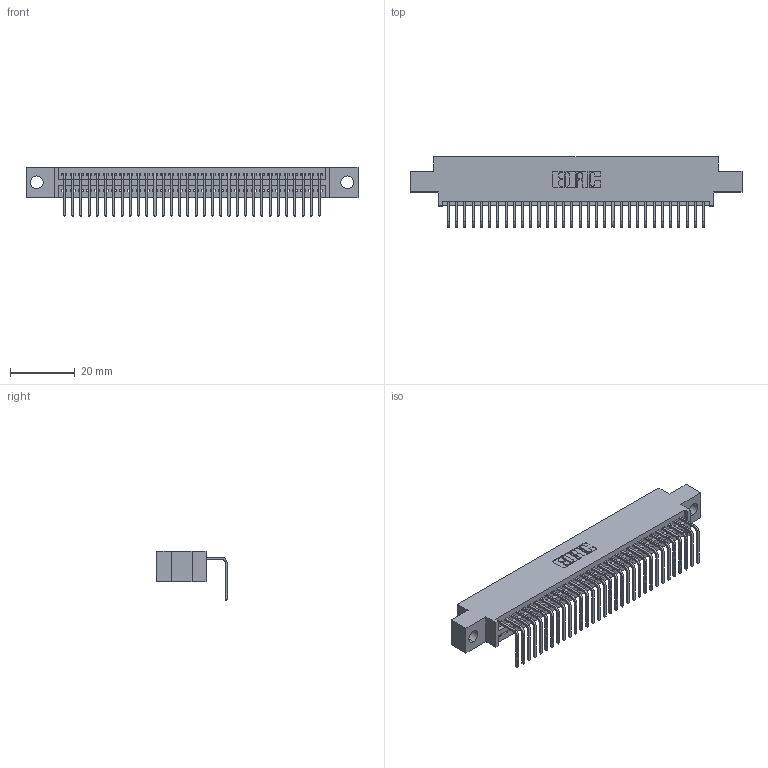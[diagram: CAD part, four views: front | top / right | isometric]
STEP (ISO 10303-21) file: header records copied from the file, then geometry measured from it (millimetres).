
FILE_DESCRIPTION (( 'STEP AP203' ), '1' );
FILE_NAME ('395-032-558-604.STEP', '2021-06-11T14:34:18', ( '' ), ( '' ), 'SwSTEP 2.0', 'SolidWorks 2020', '' );
FILE_SCHEMA (( 'CONFIG_CONTROL_DESIGN' ));
Length unit declared in the file: inch
Products named in the file (3): 395-032-558-604; 345 Part_0.170 Offset - 0.156 Dia-TI; 345-292-001_558 Tail - 2
Assembly tree (33 placements, depth 2):
  395-032-558-604
    345 Part_0.170 Offset - 0.156 Dia-TI
    345-292-001_558 Tail - 2  x32
Bounding box: 102.49 x 21.83 x 15.37 mm (x, y, z)
Volume: 9539.9 mm3; surface area: 13137.2 mm2
Topology: 33 solids, 33 shells, 2064 faces, 6213 edges, 4098 vertices
Faces by surface type: plane 1442, cylinder 622
Entity records: 26065 total; most frequent: CARTESIAN_POINT 4526, ORIENTED_EDGE 4490, DIRECTION 3965, EDGE_CURVE 2245, LINE 1985, VECTOR 1985, VERTEX_POINT 1494, AXIS2_PLACEMENT_3D 990
